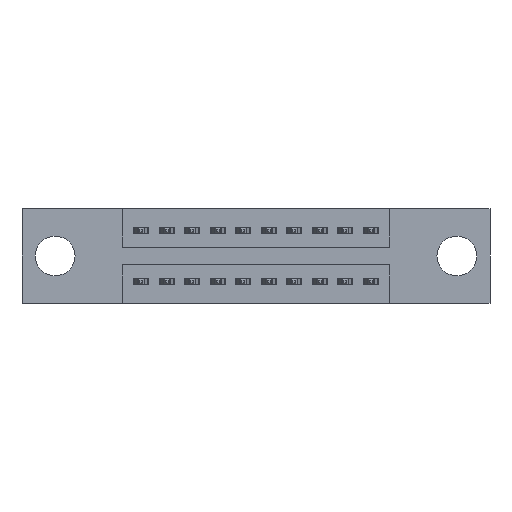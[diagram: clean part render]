
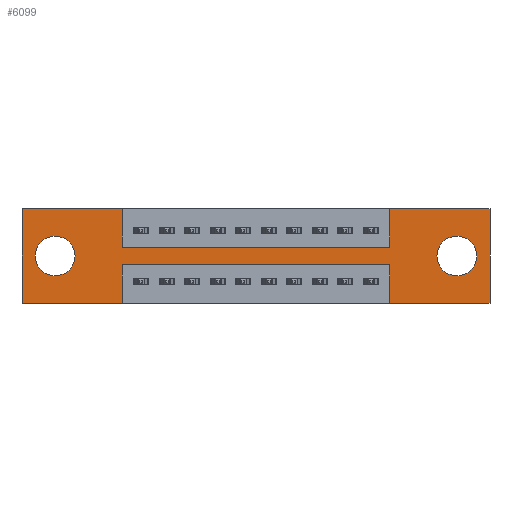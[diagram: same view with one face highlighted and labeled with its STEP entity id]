
A CAD part, front view. The second image highlights one B-rep face of the part: STEP entity #6099.
In plain terms, the highlighted planar face has unit normal (0, -1, 0).
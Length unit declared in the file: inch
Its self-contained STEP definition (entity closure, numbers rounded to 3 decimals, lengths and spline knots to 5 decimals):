
#4 = LINE ( 'NONE', #11035, #3997 ) ;
#6 = CARTESIAN_POINT ( 'NONE',  ( 0.3925, 0., -0.22 ) ) ;
#18 = AXIS2_PLACEMENT_3D ( 'NONE', #6376, #8426, #9386 ) ;
#84 = EDGE_CURVE ( 'NONE', #4117, #451, #11561, .T. ) ;
#150 = EDGE_CURVE ( 'NONE', #5583, #3042, #2729, .T. ) ;
#389 = ORIENTED_EDGE ( 'NONE', *, *, #11609, .F. ) ;
#451 = VERTEX_POINT ( 'NONE', #9524 ) ;
#784 = CIRCLE ( 'NONE', #8055, 0.078 ) ;
#851 = VERTEX_POINT ( 'NONE', #7383 ) ;
#979 = CARTESIAN_POINT ( 'NONE',  ( 0.3925, 0., 0. ) ) ;
#1072 = DIRECTION ( 'NONE',  ( 0., 0., 1. ) ) ;
#1135 = VERTEX_POINT ( 'NONE', #4212 ) ;
#1214 = CARTESIAN_POINT ( 'NONE',  ( 0.13, 0., -0.263 ) ) ;
#1290 = ORIENTED_EDGE ( 'NONE', *, *, #2054, .F. ) ;
#1304 = EDGE_CURVE ( 'NONE', #451, #7247, #11842, .T. ) ;
#1374 = VERTEX_POINT ( 'NONE', #3735 ) ;
#1383 = CARTESIAN_POINT ( 'NONE',  ( 0., 0., 0. ) ) ;
#1405 = DIRECTION ( 'NONE',  ( 0., 0., 1. ) ) ;
#1514 = EDGE_LOOP ( 'NONE', ( #4022, #6832 ) ) ;
#1649 = DIRECTION ( 'NONE',  ( 0., 1., 0. ) ) ;
#1665 = ORIENTED_EDGE ( 'NONE', *, *, #9056, .F. ) ;
#2014 = EDGE_CURVE ( 'NONE', #10143, #3263, #784, .T. ) ;
#2054 = EDGE_CURVE ( 'NONE', #7247, #5256, #4915, .T. ) ;
#2107 = DIRECTION ( 'NONE',  ( 0., 0., 1. ) ) ;
#2318 = VERTEX_POINT ( 'NONE', #5442 ) ;
#2355 = ORIENTED_EDGE ( 'NONE', *, *, #3178, .T. ) ;
#2534 = EDGE_LOOP ( 'NONE', ( #2355, #5237 ) ) ;
#2729 = LINE ( 'NONE', #3089, #9392 ) ;
#2836 = VECTOR ( 'NONE', #8337, 39.37008 ) ;
#2901 = DIRECTION ( 'NONE',  ( 0., 0., -1. ) ) ;
#2973 = ORIENTED_EDGE ( 'NONE', *, *, #150, .F. ) ;
#3019 = EDGE_LOOP ( 'NONE', ( #3307, #4886, #389, #5307, #11860, #11143, #1665, #2973, #10525, #1290, #3525, #6244 ) ) ;
#3042 = VERTEX_POINT ( 'NONE', #8556 ) ;
#3089 = CARTESIAN_POINT ( 'NONE',  ( 0.3925, 0., -0.15 ) ) ;
#3178 = EDGE_CURVE ( 'NONE', #3263, #10143, #6221, .T. ) ;
#3263 = VERTEX_POINT ( 'NONE', #7828 ) ;
#3265 = CARTESIAN_POINT ( 'NONE',  ( 0.13, 0., -0.185 ) ) ;
#3307 = ORIENTED_EDGE ( 'NONE', *, *, #8301, .F. ) ;
#3525 = ORIENTED_EDGE ( 'NONE', *, *, #1304, .F. ) ;
#3666 = LINE ( 'NONE', #6, #12060 ) ;
#3735 = CARTESIAN_POINT ( 'NONE',  ( 1.4425, 0., -0.22 ) ) ;
#3949 = DIRECTION ( 'NONE',  ( 0., 1., 0. ) ) ;
#3978 = DIRECTION ( 'NONE',  ( 0., 0., -1. ) ) ;
#3997 = VECTOR ( 'NONE', #9288, 39.37008 ) ;
#4013 = EDGE_CURVE ( 'NONE', #5256, #5583, #9504, .T. ) ;
#4022 = ORIENTED_EDGE ( 'NONE', *, *, #8198, .T. ) ;
#4025 = LINE ( 'NONE', #11551, #6199 ) ;
#4117 = VERTEX_POINT ( 'NONE', #5802 ) ;
#4171 = CARTESIAN_POINT ( 'NONE',  ( 0., 0., -0.37 ) ) ;
#4212 = CARTESIAN_POINT ( 'NONE',  ( 1.4425, 0., 0. ) ) ;
#4215 = DIRECTION ( 'NONE',  ( -1., 0., 0. ) ) ;
#4445 = CARTESIAN_POINT ( 'NONE',  ( 0., 0., 0. ) ) ;
#4609 = CARTESIAN_POINT ( 'NONE',  ( 0., 0., 0. ) ) ;
#4862 = CARTESIAN_POINT ( 'NONE',  ( 1.4425, 0., -0.37 ) ) ;
#4886 = ORIENTED_EDGE ( 'NONE', *, *, #11485, .F. ) ;
#4915 = LINE ( 'NONE', #1383, #8760 ) ;
#5036 = LINE ( 'NONE', #4445, #2836 ) ;
#5186 = VECTOR ( 'NONE', #9599, 39.37008 ) ;
#5237 = ORIENTED_EDGE ( 'NONE', *, *, #2014, .T. ) ;
#5256 = VERTEX_POINT ( 'NONE', #979 ) ;
#5307 = ORIENTED_EDGE ( 'NONE', *, *, #7368, .F. ) ;
#5349 = AXIS2_PLACEMENT_3D ( 'NONE', #10953, #1649, #2901 ) ;
#5442 = CARTESIAN_POINT ( 'NONE',  ( 1.705, 0., -0.107 ) ) ;
#5583 = VERTEX_POINT ( 'NONE', #8594 ) ;
#5585 = FACE_OUTER_BOUND ( 'NONE', #3019, .T. ) ;
#5802 = CARTESIAN_POINT ( 'NONE',  ( 0.3925, 0., -0.37 ) ) ;
#5817 = CIRCLE ( 'NONE', #5349, 0.078 ) ;
#5830 = VERTEX_POINT ( 'NONE', #10487 ) ;
#6099 = ADVANCED_FACE ( 'NONE', ( #8109, #7204, #5585 ), #7391, .T. ) ;
#6199 = VECTOR ( 'NONE', #1072, 39.37008 ) ;
#6221 = CIRCLE ( 'NONE', #9642, 0.078 ) ;
#6244 = ORIENTED_EDGE ( 'NONE', *, *, #84, .F. ) ;
#6376 = CARTESIAN_POINT ( 'NONE',  ( 0., 0., -0.37 ) ) ;
#6615 = VERTEX_POINT ( 'NONE', #10250 ) ;
#6680 = VECTOR ( 'NONE', #1405, 39.37008 ) ;
#6726 = DIRECTION ( 'NONE',  ( -1., 0., 0. ) ) ;
#6755 = DIRECTION ( 'NONE',  ( 0., 1., 0. ) ) ;
#6803 = DIRECTION ( 'NONE',  ( 1., 0., 0. ) ) ;
#6832 = ORIENTED_EDGE ( 'NONE', *, *, #10856, .T. ) ;
#7202 = VERTEX_POINT ( 'NONE', #8531 ) ;
#7204 = FACE_BOUND ( 'NONE', #2534, .T. ) ;
#7247 = VERTEX_POINT ( 'NONE', #4609 ) ;
#7368 = EDGE_CURVE ( 'NONE', #851, #6615, #9551, .T. ) ;
#7383 = CARTESIAN_POINT ( 'NONE',  ( 1.835, 0., -0.37 ) ) ;
#7391 = PLANE ( 'NONE',  #18 ) ;
#7784 = CARTESIAN_POINT ( 'NONE',  ( 0., 0., -0.37 ) ) ;
#7806 = EDGE_CURVE ( 'NONE', #7202, #851, #10817, .T. ) ;
#7828 = CARTESIAN_POINT ( 'NONE',  ( 0.13, 0., -0.107 ) ) ;
#8055 = AXIS2_PLACEMENT_3D ( 'NONE', #9603, #3949, #10500 ) ;
#8109 = FACE_BOUND ( 'NONE', #1514, .T. ) ;
#8198 = EDGE_CURVE ( 'NONE', #2318, #11699, #5817, .T. ) ;
#8301 = EDGE_CURVE ( 'NONE', #5830, #4117, #4, .T. ) ;
#8337 = DIRECTION ( 'NONE',  ( 1., 0., 0. ) ) ;
#8422 = DIRECTION ( 'NONE',  ( -1., 0., 0. ) ) ;
#8426 = DIRECTION ( 'NONE',  ( 0., -1., 0. ) ) ;
#8502 = VECTOR ( 'NONE', #10533, 39.37008 ) ;
#8531 = CARTESIAN_POINT ( 'NONE',  ( 1.835, 0., 0. ) ) ;
#8556 = CARTESIAN_POINT ( 'NONE',  ( 1.4425, 0., -0.15 ) ) ;
#8594 = CARTESIAN_POINT ( 'NONE',  ( 0.3925, 0., -0.15 ) ) ;
#8645 = CARTESIAN_POINT ( 'NONE',  ( 1.835, 0., 0. ) ) ;
#8701 = EDGE_CURVE ( 'NONE', #1135, #7202, #5036, .T. ) ;
#8760 = VECTOR ( 'NONE', #11591, 39.37008 ) ;
#8880 = DIRECTION ( 'NONE',  ( 0., 1., 0. ) ) ;
#8952 = CARTESIAN_POINT ( 'NONE',  ( 0., 0., 0. ) ) ;
#9056 = EDGE_CURVE ( 'NONE', #3042, #1135, #4025, .T. ) ;
#9103 = VECTOR ( 'NONE', #6726, 39.37008 ) ;
#9288 = DIRECTION ( 'NONE',  ( 0., 0., -1. ) ) ;
#9386 = DIRECTION ( 'NONE',  ( 0., 0., -1. ) ) ;
#9392 = VECTOR ( 'NONE', #6803, 39.37008 ) ;
#9432 = AXIS2_PLACEMENT_3D ( 'NONE', #9592, #6755, #3978 ) ;
#9504 = LINE ( 'NONE', #10447, #5186 ) ;
#9524 = CARTESIAN_POINT ( 'NONE',  ( 0., 0., -0.37 ) ) ;
#9551 = LINE ( 'NONE', #7784, #9103 ) ;
#9592 = CARTESIAN_POINT ( 'NONE',  ( 1.705, 0., -0.185 ) ) ;
#9599 = DIRECTION ( 'NONE',  ( 0., 0., -1. ) ) ;
#9603 = CARTESIAN_POINT ( 'NONE',  ( 0.13, 0., -0.185 ) ) ;
#9642 = AXIS2_PLACEMENT_3D ( 'NONE', #3265, #8880, #11700 ) ;
#10143 = VERTEX_POINT ( 'NONE', #1214 ) ;
#10250 = CARTESIAN_POINT ( 'NONE',  ( 1.4425, 0., -0.37 ) ) ;
#10447 = CARTESIAN_POINT ( 'NONE',  ( 0.3925, 0., 0. ) ) ;
#10487 = CARTESIAN_POINT ( 'NONE',  ( 0.3925, 0., -0.22 ) ) ;
#10500 = DIRECTION ( 'NONE',  ( 0., 0., 1. ) ) ;
#10525 = ORIENTED_EDGE ( 'NONE', *, *, #4013, .F. ) ;
#10533 = DIRECTION ( 'NONE',  ( 0., 0., -1. ) ) ;
#10571 = VECTOR ( 'NONE', #2107, 39.37008 ) ;
#10817 = LINE ( 'NONE', #8645, #8502 ) ;
#10856 = EDGE_CURVE ( 'NONE', #11699, #2318, #11336, .T. ) ;
#10953 = CARTESIAN_POINT ( 'NONE',  ( 1.705, 0., -0.185 ) ) ;
#11035 = CARTESIAN_POINT ( 'NONE',  ( 0.3925, 0., -0.37 ) ) ;
#11143 = ORIENTED_EDGE ( 'NONE', *, *, #8701, .F. ) ;
#11268 = VECTOR ( 'NONE', #4215, 39.37008 ) ;
#11336 = CIRCLE ( 'NONE', #9432, 0.078 ) ;
#11392 = CARTESIAN_POINT ( 'NONE',  ( 1.705, 0., -0.263 ) ) ;
#11475 = LINE ( 'NONE', #4862, #10571 ) ;
#11485 = EDGE_CURVE ( 'NONE', #1374, #5830, #3666, .T. ) ;
#11551 = CARTESIAN_POINT ( 'NONE',  ( 1.4425, 0., 0. ) ) ;
#11561 = LINE ( 'NONE', #4171, #11268 ) ;
#11591 = DIRECTION ( 'NONE',  ( 1., 0., 0. ) ) ;
#11609 = EDGE_CURVE ( 'NONE', #6615, #1374, #11475, .T. ) ;
#11699 = VERTEX_POINT ( 'NONE', #11392 ) ;
#11700 = DIRECTION ( 'NONE',  ( 0., 0., 1. ) ) ;
#11842 = LINE ( 'NONE', #8952, #6680 ) ;
#11860 = ORIENTED_EDGE ( 'NONE', *, *, #7806, .F. ) ;
#12060 = VECTOR ( 'NONE', #8422, 39.37008 ) ;
